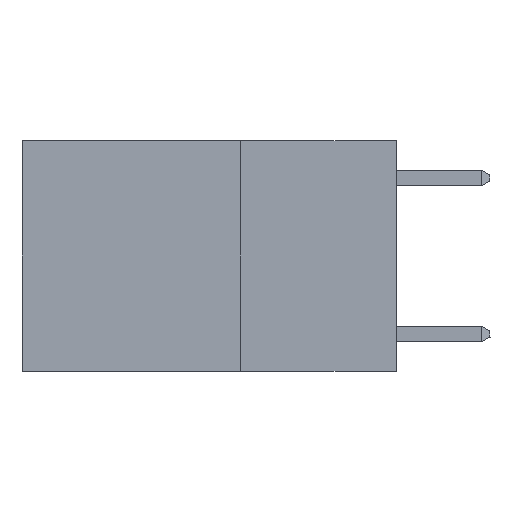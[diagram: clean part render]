
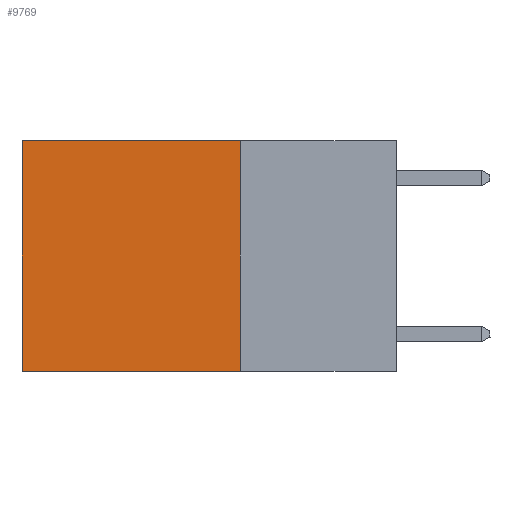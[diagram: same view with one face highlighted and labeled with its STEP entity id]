
A CAD part, left-side view. The second image highlights one B-rep face of the part: STEP entity #9769.
In plain terms, the highlighted planar face has unit normal (-1, 0, 0).
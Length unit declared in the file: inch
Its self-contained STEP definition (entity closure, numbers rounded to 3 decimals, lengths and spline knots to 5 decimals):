
#56 = CARTESIAN_POINT ( 'NONE',  ( 0.2625, 0.25, 0. ) ) ;
#804 = EDGE_CURVE ( 'NONE', #7236, #2462, #8232, .T. ) ;
#1102 = CARTESIAN_POINT ( 'NONE',  ( 0.2625, 0.25, -0.37 ) ) ;
#1104 = DIRECTION ( 'NONE',  ( 0., 0., -1. ) ) ;
#1168 = DIRECTION ( 'NONE',  ( 1., 0., 0. ) ) ;
#1300 = FACE_OUTER_BOUND ( 'NONE', #3232, .T. ) ;
#2067 = EDGE_CURVE ( 'NONE', #2462, #4741, #5217, .T. ) ;
#2128 = AXIS2_PLACEMENT_3D ( 'NONE', #56, #1168, #7014 ) ;
#2462 = VERTEX_POINT ( 'NONE', #1102 ) ;
#2935 = CARTESIAN_POINT ( 'NONE',  ( 0.2625, 0.25, -0.37 ) ) ;
#3040 = CARTESIAN_POINT ( 'NONE',  ( 0.2625, 0.6, 0. ) ) ;
#3232 = EDGE_LOOP ( 'NONE', ( #6510, #6478, #5260, #5877 ) ) ;
#3553 = VECTOR ( 'NONE', #9451, 39.37008 ) ;
#4741 = VERTEX_POINT ( 'NONE', #7687 ) ;
#5186 = LINE ( 'NONE', #10665, #8870 ) ;
#5217 = LINE ( 'NONE', #2935, #7081 ) ;
#5260 = ORIENTED_EDGE ( 'NONE', *, *, #804, .F. ) ;
#5318 = DIRECTION ( 'NONE',  ( 0., 1., 0. ) ) ;
#5877 = ORIENTED_EDGE ( 'NONE', *, *, #8734, .T. ) ;
#6478 = ORIENTED_EDGE ( 'NONE', *, *, #2067, .F. ) ;
#6510 = ORIENTED_EDGE ( 'NONE', *, *, #10531, .T. ) ;
#7014 = DIRECTION ( 'NONE',  ( 0., 0., -1. ) ) ;
#7081 = VECTOR ( 'NONE', #5318, 39.37008 ) ;
#7236 = VERTEX_POINT ( 'NONE', #8168 ) ;
#7687 = CARTESIAN_POINT ( 'NONE',  ( 0.2625, 0.6, -0.37 ) ) ;
#8168 = CARTESIAN_POINT ( 'NONE',  ( 0.2625, 0.25, 0. ) ) ;
#8232 = LINE ( 'NONE', #9538, #3553 ) ;
#8384 = DIRECTION ( 'NONE',  ( 0., 1., 0. ) ) ;
#8734 = EDGE_CURVE ( 'NONE', #7236, #9118, #5186, .T. ) ;
#8870 = VECTOR ( 'NONE', #8384, 39.37008 ) ;
#9118 = VERTEX_POINT ( 'NONE', #9580 ) ;
#9308 = PLANE ( 'NONE',  #2128 ) ;
#9451 = DIRECTION ( 'NONE',  ( 0., 0., -1. ) ) ;
#9538 = CARTESIAN_POINT ( 'NONE',  ( 0.2625, 0.25, 0. ) ) ;
#9540 = VECTOR ( 'NONE', #1104, 39.37008 ) ;
#9580 = CARTESIAN_POINT ( 'NONE',  ( 0.2625, 0.6, 0. ) ) ;
#9768 = LINE ( 'NONE', #3040, #9540 ) ;
#9769 = ADVANCED_FACE ( 'NONE', ( #1300 ), #9308, .F. ) ;
#10531 = EDGE_CURVE ( 'NONE', #9118, #4741, #9768, .T. ) ;
#10665 = CARTESIAN_POINT ( 'NONE',  ( 0.2625, 0.25, 0. ) ) ;
